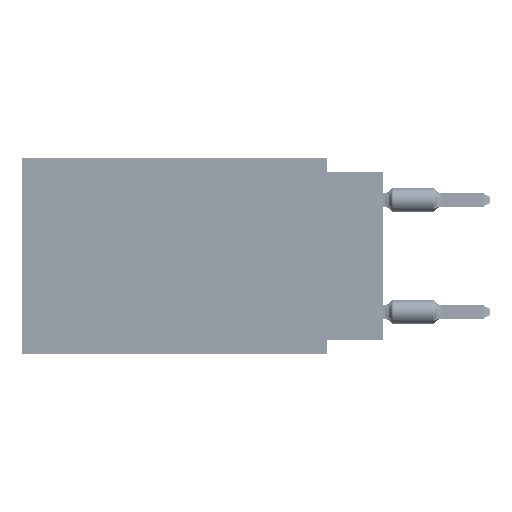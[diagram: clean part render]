
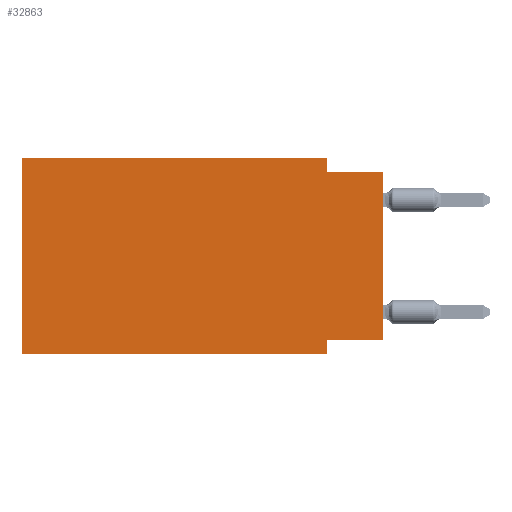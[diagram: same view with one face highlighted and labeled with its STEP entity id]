
A CAD part, left-side view. The second image highlights one B-rep face of the part: STEP entity #32863.
In plain terms, the highlighted planar face has unit normal (-1, 0, 0).
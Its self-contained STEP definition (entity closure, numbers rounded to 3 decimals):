
#1304 = CARTESIAN_POINT ( 'NONE',  ( 0., 16.383, -8.89 ) ) ;
#2041 = VECTOR ( 'NONE', #9612, 1000. ) ;
#2094 = CARTESIAN_POINT ( 'NONE',  ( 0., 16.383, 0. ) ) ;
#5409 = VERTEX_POINT ( 'NONE', #7381 ) ;
#7381 = CARTESIAN_POINT ( 'NONE',  ( 0., 0., -0.635 ) ) ;
#7553 = ORIENTED_EDGE ( 'NONE', *, *, #75114, .F. ) ;
#8674 = DIRECTION ( 'NONE',  ( 0., 0., -1. ) ) ;
#9612 = DIRECTION ( 'NONE',  ( 0., -1., 0. ) ) ;
#12569 = DIRECTION ( 'NONE',  ( 0., -1., 0. ) ) ;
#12631 = LINE ( 'NONE', #39290, #61812 ) ;
#15278 = VERTEX_POINT ( 'NONE', #20198 ) ;
#15423 = CARTESIAN_POINT ( 'NONE',  ( 0., 0., -8.255 ) ) ;
#16822 = DIRECTION ( 'NONE',  ( 0., 0., -1. ) ) ;
#17252 = DIRECTION ( 'NONE',  ( 1., 0., 0. ) ) ;
#17690 = FACE_OUTER_BOUND ( 'NONE', #43317, .T. ) ;
#19638 = EDGE_CURVE ( 'NONE', #69500, #41699, #54191, .T. ) ;
#20198 = CARTESIAN_POINT ( 'NONE',  ( 0., 2.54, -0.635 ) ) ;
#21153 = EDGE_CURVE ( 'NONE', #69500, #86533, #46234, .T. ) ;
#21296 = LINE ( 'NONE', #47959, #49362 ) ;
#24092 = CARTESIAN_POINT ( 'NONE',  ( 0., 16.383, 0. ) ) ;
#28621 = EDGE_CURVE ( 'NONE', #15278, #5409, #83684, .T. ) ;
#32237 = CARTESIAN_POINT ( 'NONE',  ( 0., 16.383, -8.89 ) ) ;
#32863 = ADVANCED_FACE ( 'NONE', ( #17690 ), #44367, .F. ) ;
#33346 = VERTEX_POINT ( 'NONE', #48742 ) ;
#34795 = VECTOR ( 'NONE', #12569, 1000. ) ;
#35097 = LINE ( 'NONE', #15423, #66309 ) ;
#36844 = DIRECTION ( 'NONE',  ( 0., -1., 0. ) ) ;
#38791 = VECTOR ( 'NONE', #81315, 1000. ) ;
#39290 = CARTESIAN_POINT ( 'NONE',  ( 0., 0., 0. ) ) ;
#41699 = VERTEX_POINT ( 'NONE', #24092 ) ;
#43317 = EDGE_LOOP ( 'NONE', ( #70021, #51501, #70922, #7553, #62181, #75294, #77356, #53850 ) ) ;
#44367 = PLANE ( 'NONE',  #53072 ) ;
#46234 = LINE ( 'NONE', #32237, #34795 ) ;
#47959 = CARTESIAN_POINT ( 'NONE',  ( 0., 2.54, 0. ) ) ;
#48491 = LINE ( 'NONE', #56353, #83983 ) ;
#48742 = CARTESIAN_POINT ( 'NONE',  ( 0., 0., -8.255 ) ) ;
#49362 = VECTOR ( 'NONE', #55821, 1000. ) ;
#50526 = VERTEX_POINT ( 'NONE', #81420 ) ;
#51501 = ORIENTED_EDGE ( 'NONE', *, *, #28621, .F. ) ;
#52877 = DIRECTION ( 'NONE',  ( 0., 0., 1. ) ) ;
#53072 = AXIS2_PLACEMENT_3D ( 'NONE', #78519, #17252, #16822 ) ;
#53850 = ORIENTED_EDGE ( 'NONE', *, *, #83610, .F. ) ;
#54149 = CARTESIAN_POINT ( 'NONE',  ( 0., 2.54, -8.89 ) ) ;
#54191 = LINE ( 'NONE', #2094, #38791 ) ;
#55680 = CARTESIAN_POINT ( 'NONE',  ( 0., 0., -0.635 ) ) ;
#55821 = DIRECTION ( 'NONE',  ( 0., 0., -1. ) ) ;
#56353 = CARTESIAN_POINT ( 'NONE',  ( 0., 2.54, -8.89 ) ) ;
#58176 = LINE ( 'NONE', #70859, #2041 ) ;
#61389 = EDGE_CURVE ( 'NONE', #50526, #15278, #21296, .T. ) ;
#61806 = DIRECTION ( 'NONE',  ( 0., 1., 0. ) ) ;
#61812 = VECTOR ( 'NONE', #52877, 1000. ) ;
#62181 = ORIENTED_EDGE ( 'NONE', *, *, #19638, .F. ) ;
#62980 = EDGE_CURVE ( 'NONE', #63568, #86533, #48491, .T. ) ;
#63568 = VERTEX_POINT ( 'NONE', #70241 ) ;
#66309 = VECTOR ( 'NONE', #61806, 1000. ) ;
#69500 = VERTEX_POINT ( 'NONE', #1304 ) ;
#70021 = ORIENTED_EDGE ( 'NONE', *, *, #72910, .T. ) ;
#70241 = CARTESIAN_POINT ( 'NONE',  ( 0., 2.54, -8.255 ) ) ;
#70859 = CARTESIAN_POINT ( 'NONE',  ( 0., 16.383, 0. ) ) ;
#70922 = ORIENTED_EDGE ( 'NONE', *, *, #61389, .F. ) ;
#72910 = EDGE_CURVE ( 'NONE', #33346, #5409, #12631, .T. ) ;
#75114 = EDGE_CURVE ( 'NONE', #41699, #50526, #58176, .T. ) ;
#75294 = ORIENTED_EDGE ( 'NONE', *, *, #21153, .T. ) ;
#77356 = ORIENTED_EDGE ( 'NONE', *, *, #62980, .F. ) ;
#78519 = CARTESIAN_POINT ( 'NONE',  ( 0., 16.383, 0. ) ) ;
#81315 = DIRECTION ( 'NONE',  ( 0., 0., 1. ) ) ;
#81420 = CARTESIAN_POINT ( 'NONE',  ( 0., 2.54, 0. ) ) ;
#83515 = VECTOR ( 'NONE', #36844, 1000. ) ;
#83610 = EDGE_CURVE ( 'NONE', #33346, #63568, #35097, .T. ) ;
#83684 = LINE ( 'NONE', #55680, #83515 ) ;
#83983 = VECTOR ( 'NONE', #8674, 1000. ) ;
#86533 = VERTEX_POINT ( 'NONE', #54149 ) ;
